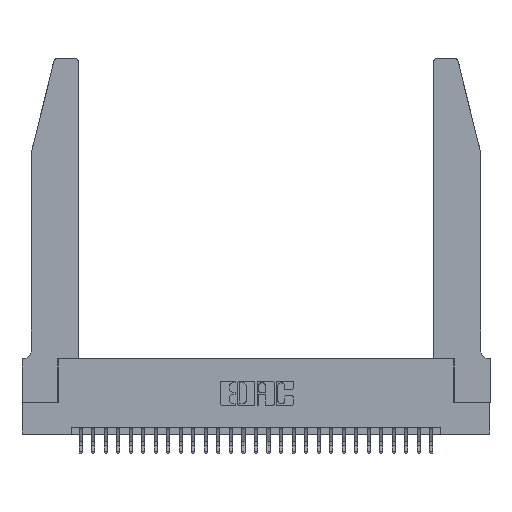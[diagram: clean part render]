
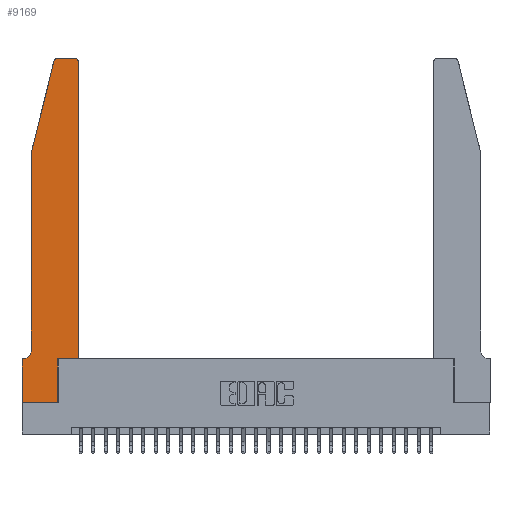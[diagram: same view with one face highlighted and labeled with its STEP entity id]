
A CAD part, top view. The second image highlights one B-rep face of the part: STEP entity #9169.
In plain terms, the highlighted planar face has unit normal (0, 0, 1).
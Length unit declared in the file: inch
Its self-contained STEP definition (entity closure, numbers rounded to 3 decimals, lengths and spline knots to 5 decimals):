
#247 = CARTESIAN_POINT ( 'NONE',  ( 0.2865, 0.35, 0.37 ) ) ;
#937 = VERTEX_POINT ( 'NONE', #247 ) ;
#1027 = VECTOR ( 'NONE', #25666, 39.37008 ) ;
#1149 = DIRECTION ( 'NONE',  ( -1., 0., 0. ) ) ;
#1374 = CARTESIAN_POINT ( 'NONE',  ( 0.0755, 2., 0.37 ) ) ;
#1498 = ORIENTED_EDGE ( 'NONE', *, *, #27426, .T. ) ;
#2962 = CARTESIAN_POINT ( 'NONE',  ( 0.0755, 2., 0.37 ) ) ;
#3518 = CARTESIAN_POINT ( 'NONE',  ( 0., 0., 0.37 ) ) ;
#3890 = ORIENTED_EDGE ( 'NONE', *, *, #15564, .T. ) ;
#3922 = CARTESIAN_POINT ( 'NONE',  ( 0.0755, 0.42, 0.37 ) ) ;
#4087 = DIRECTION ( 'NONE',  ( 1., 0., 0. ) ) ;
#4221 = CARTESIAN_POINT ( 'NONE',  ( 0., 0.35, 0.37 ) ) ;
#4236 = EDGE_CURVE ( 'NONE', #17975, #11951, #17019, .T. ) ;
#4290 = CARTESIAN_POINT ( 'NONE',  ( 0., 0., 0.37 ) ) ;
#4368 = VERTEX_POINT ( 'NONE', #8874 ) ;
#4608 = DIRECTION ( 'NONE',  ( 1., 0., 0. ) ) ;
#4825 = DIRECTION ( 'NONE',  ( -1., 0., 0. ) ) ;
#5288 = VERTEX_POINT ( 'NONE', #20399 ) ;
#5888 = LINE ( 'NONE', #27390, #9768 ) ;
#6094 = CARTESIAN_POINT ( 'NONE',  ( 0.284, 2.75, 0.37 ) ) ;
#6128 = CARTESIAN_POINT ( 'NONE',  ( 0.4505, 0.35, 0.37 ) ) ;
#6366 = ORIENTED_EDGE ( 'NONE', *, *, #14538, .T. ) ;
#6446 = ORIENTED_EDGE ( 'NONE', *, *, #18319, .T. ) ;
#7059 = LINE ( 'NONE', #16376, #1027 ) ;
#7542 = VECTOR ( 'NONE', #8086, 39.37008 ) ;
#7662 = VERTEX_POINT ( 'NONE', #3922 ) ;
#7860 = EDGE_CURVE ( 'NONE', #4368, #17933, #15382, .T. ) ;
#8086 = DIRECTION ( 'NONE',  ( 0., -1., 0. ) ) ;
#8124 = EDGE_CURVE ( 'NONE', #7662, #12308, #14696, .T. ) ;
#8613 = ORIENTED_EDGE ( 'NONE', *, *, #8124, .T. ) ;
#8645 = EDGE_CURVE ( 'NONE', #19713, #17975, #17468, .T. ) ;
#8874 = CARTESIAN_POINT ( 'NONE',  ( 0.4205, 2.75, 0.37 ) ) ;
#8875 = DIRECTION ( 'NONE',  ( 0., 0., 1. ) ) ;
#8876 = CARTESIAN_POINT ( 'NONE',  ( 0.2605, 2.75, 0.37 ) ) ;
#9169 = ADVANCED_FACE ( 'NONE', ( #26067 ), #23282, .T. ) ;
#9601 = CARTESIAN_POINT ( 'NONE',  ( 0.4505, 2.72, 0.37 ) ) ;
#9768 = VECTOR ( 'NONE', #25387, 39.37008 ) ;
#9794 = CARTESIAN_POINT ( 'NONE',  ( 0.0055, 0.35, 0.37 ) ) ;
#9820 = DIRECTION ( 'NONE',  ( 0., 0., 1. ) ) ;
#9872 = VECTOR ( 'NONE', #17175, 39.37008 ) ;
#10022 = VECTOR ( 'NONE', #4825, 39.37008 ) ;
#10084 = DIRECTION ( 'NONE',  ( 1., 0., 0. ) ) ;
#10100 = DIRECTION ( 'NONE',  ( 1., 0., 0. ) ) ;
#10689 = VECTOR ( 'NONE', #29495, 39.37008 ) ;
#11068 = LINE ( 'NONE', #13745, #10689 ) ;
#11235 = ORIENTED_EDGE ( 'NONE', *, *, #14675, .T. ) ;
#11831 = ORIENTED_EDGE ( 'NONE', *, *, #4236, .T. ) ;
#11951 = VERTEX_POINT ( 'NONE', #17134 ) ;
#12217 = AXIS2_PLACEMENT_3D ( 'NONE', #27178, #18261, #10084 ) ;
#12266 = CARTESIAN_POINT ( 'NONE',  ( 0.4505, 0.35, 0.37 ) ) ;
#12308 = VERTEX_POINT ( 'NONE', #9794 ) ;
#12598 = CARTESIAN_POINT ( 'NONE',  ( 0.0755, 0.35, 0.37 ) ) ;
#12837 = VERTEX_POINT ( 'NONE', #2962 ) ;
#13212 = AXIS2_PLACEMENT_3D ( 'NONE', #23506, #9820, #10100 ) ;
#13606 = ORIENTED_EDGE ( 'NONE', *, *, #25273, .T. ) ;
#13745 = CARTESIAN_POINT ( 'NONE',  ( 0.0755, 2., 0.37 ) ) ;
#14538 = EDGE_CURVE ( 'NONE', #17933, #5288, #18435, .T. ) ;
#14675 = EDGE_CURVE ( 'NONE', #11951, #937, #7059, .T. ) ;
#14696 = CIRCLE ( 'NONE', #27039, 0.07 ) ;
#15097 = CARTESIAN_POINT ( 'NONE',  ( 0., 0.35, 0.37 ) ) ;
#15382 = LINE ( 'NONE', #8876, #10022 ) ;
#15564 = EDGE_CURVE ( 'NONE', #937, #26774, #23768, .T. ) ;
#15780 = ORIENTED_EDGE ( 'NONE', *, *, #7860, .T. ) ;
#16376 = CARTESIAN_POINT ( 'NONE',  ( 0.2865, 0.35, 0.37 ) ) ;
#16974 = VECTOR ( 'NONE', #4608, 39.37008 ) ;
#17019 = LINE ( 'NONE', #27745, #27744 ) ;
#17124 = VECTOR ( 'NONE', #21659, 39.37008 ) ;
#17134 = CARTESIAN_POINT ( 'NONE',  ( 0.2865, 0., 0.37 ) ) ;
#17175 = DIRECTION ( 'NONE',  ( -1., 0., 0. ) ) ;
#17468 = LINE ( 'NONE', #3518, #7542 ) ;
#17818 = AXIS2_PLACEMENT_3D ( 'NONE', #4221, #8875, #4087 ) ;
#17933 = VERTEX_POINT ( 'NONE', #6094 ) ;
#17975 = VERTEX_POINT ( 'NONE', #4290 ) ;
#18261 = DIRECTION ( 'NONE',  ( 0., 0., 1. ) ) ;
#18319 = EDGE_CURVE ( 'NONE', #22061, #4368, #20164, .T. ) ;
#18435 = CIRCLE ( 'NONE', #12217, 0.03 ) ;
#19133 = DIRECTION ( 'NONE',  ( 0., 0., -1. ) ) ;
#19713 = VERTEX_POINT ( 'NONE', #15097 ) ;
#20164 = CIRCLE ( 'NONE', #13212, 0.03 ) ;
#20399 = CARTESIAN_POINT ( 'NONE',  ( 0.25487, 2.72718, 0.37 ) ) ;
#21082 = EDGE_CURVE ( 'NONE', #12837, #7662, #11068, .T. ) ;
#21659 = DIRECTION ( 'NONE',  ( -0.239, -0.971, 0. ) ) ;
#22061 = VERTEX_POINT ( 'NONE', #9601 ) ;
#23092 = LINE ( 'NONE', #12598, #9872 ) ;
#23213 = LINE ( 'NONE', #1374, #17124 ) ;
#23282 = PLANE ( 'NONE',  #17818 ) ;
#23506 = CARTESIAN_POINT ( 'NONE',  ( 0.4205, 2.72, 0.37 ) ) ;
#23755 = EDGE_CURVE ( 'NONE', #12308, #19713, #23092, .T. ) ;
#23768 = LINE ( 'NONE', #6128, #16974 ) ;
#25273 = EDGE_CURVE ( 'NONE', #26774, #22061, #5888, .T. ) ;
#25387 = DIRECTION ( 'NONE',  ( 0., 1., 0. ) ) ;
#25543 = DIRECTION ( 'NONE',  ( 1., 0., 0. ) ) ;
#25666 = DIRECTION ( 'NONE',  ( 0., 1., 0. ) ) ;
#26067 = FACE_OUTER_BOUND ( 'NONE', #26892, .T. ) ;
#26118 = ORIENTED_EDGE ( 'NONE', *, *, #23755, .T. ) ;
#26774 = VERTEX_POINT ( 'NONE', #12266 ) ;
#26892 = EDGE_LOOP ( 'NONE', ( #15780, #6366, #1498, #28546, #8613, #26118, #27013, #11831, #11235, #3890, #13606, #6446 ) ) ;
#27013 = ORIENTED_EDGE ( 'NONE', *, *, #8645, .T. ) ;
#27039 = AXIS2_PLACEMENT_3D ( 'NONE', #27646, #19133, #1149 ) ;
#27178 = CARTESIAN_POINT ( 'NONE',  ( 0.284, 2.72, 0.37 ) ) ;
#27390 = CARTESIAN_POINT ( 'NONE',  ( 0.4505, 0.35, 0.37 ) ) ;
#27426 = EDGE_CURVE ( 'NONE', #5288, #12837, #23213, .T. ) ;
#27646 = CARTESIAN_POINT ( 'NONE',  ( 0.0055, 0.42, 0.37 ) ) ;
#27744 = VECTOR ( 'NONE', #25543, 39.37008 ) ;
#27745 = CARTESIAN_POINT ( 'NONE',  ( 0., 0., 0.37 ) ) ;
#28546 = ORIENTED_EDGE ( 'NONE', *, *, #21082, .T. ) ;
#29495 = DIRECTION ( 'NONE',  ( 0., -1., 0. ) ) ;
